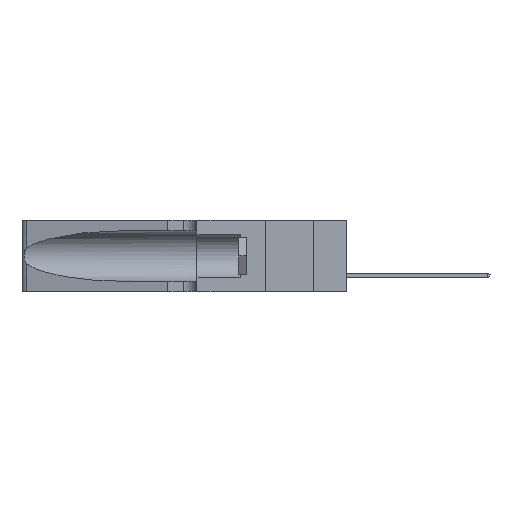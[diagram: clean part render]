
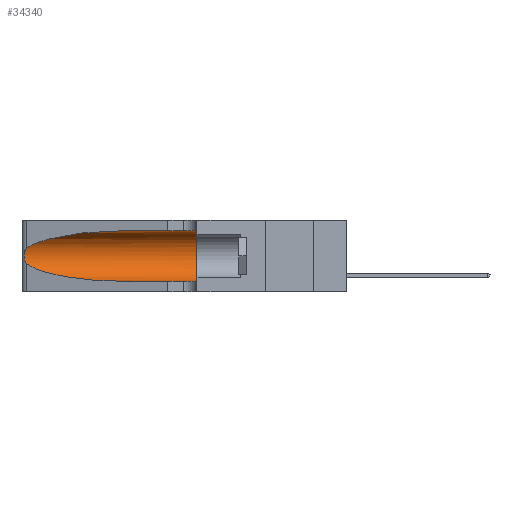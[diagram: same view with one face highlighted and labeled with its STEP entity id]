
A CAD part, left-side view. The second image highlights one B-rep face of the part: STEP entity #34340.
In plain terms, the highlighted cylindrical face has radius 3.308 mm (diameter 6.617 mm), a partial arc.
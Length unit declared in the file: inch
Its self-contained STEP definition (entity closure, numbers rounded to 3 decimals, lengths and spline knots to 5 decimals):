
#323 = EDGE_CURVE ( 'NONE', #18879, #18851, #22355, .T. ) ;
#1879 = ORIENTED_EDGE ( 'NONE', *, *, #11291, .F. ) ;
#2543 = CARTESIAN_POINT ( 'NONE',  ( 0.25555, 1.22993, 0.14849 ) ) ;
#2659 = CARTESIAN_POINT ( 'NONE',  ( 0.2373, 1.15595, 0.08982 ) ) ;
#2706 = CARTESIAN_POINT ( 'NONE',  ( 0.25487, 1.22718, 0.22369 ) ) ;
#3134 = VERTEX_POINT ( 'NONE', #41713 ) ;
#4005 = EDGE_CURVE ( 'NONE', #18851, #28390, #4882, .T. ) ;
#4381 = CARTESIAN_POINT ( 'NONE',  ( 0.26075, 1.23896, 0.178 ) ) ;
#4882 =( BOUNDED_CURVE ( )  B_SPLINE_CURVE ( 3, ( #34687, #2659, #30677, #18717 ),
 .UNSPECIFIED., .F., .F. ) 
 B_SPLINE_CURVE_WITH_KNOTS ( ( 4, 4 ),
 ( 3.44316, 4.71239 ),
 .UNSPECIFIED. ) 
 CURVE ( )  GEOMETRIC_REPRESENTATION_ITEM ( )  RATIONAL_B_SPLINE_CURVE ( ( 1., 0.87, 0.87, 1. ) ) 
 REPRESENTATION_ITEM ( '' )  );
#5112 = LINE ( 'NONE', #31419, #37330 ) ;
#6915 = ORIENTED_EDGE ( 'NONE', *, *, #20891, .T. ) ;
#7603 = CARTESIAN_POINT ( 'NONE',  ( 0.25487, 1.22718, 0.22369 ) ) ;
#7993 = CARTESIAN_POINT ( 'NONE',  ( 0.1305, 1.61858, 0.31525 ) ) ;
#11291 = EDGE_CURVE ( 'NONE', #23974, #41433, #17209, .T. ) ;
#12127 = FACE_OUTER_BOUND ( 'NONE', #50442, .T. ) ;
#14877 = CARTESIAN_POINT ( 'NONE',  ( 0.1305, 0.35, 0.31525 ) ) ;
#15118 = CARTESIAN_POINT ( 'NONE',  ( 0.1305, 0.72297, 0.05475 ) ) ;
#16790 = CARTESIAN_POINT ( 'NONE',  ( 0.26017, 1.23833, 0.17102 ) ) ;
#16837 = EDGE_CURVE ( 'NONE', #3134, #23974, #25311, .T. ) ;
#17209 = CIRCLE ( 'NONE', #35773, 0.13025 ) ;
#18717 = CARTESIAN_POINT ( 'NONE',  ( 0.1305, 0.72297, 0.05475 ) ) ;
#18851 = VERTEX_POINT ( 'NONE', #25180 ) ;
#18879 = VERTEX_POINT ( 'NONE', #41103 ) ;
#19091 = CARTESIAN_POINT ( 'NONE',  ( 0.26075, 1.23896, 0.19203 ) ) ;
#19130 = VECTOR ( 'NONE', #39382, 39.37008 ) ;
#19698 = DIRECTION ( 'NONE',  ( 0., -1., 0. ) ) ;
#20891 = EDGE_CURVE ( 'NONE', #28390, #41433, #5112, .T. ) ;
#21213 = DIRECTION ( 'NONE',  ( 0., 0., 1. ) ) ;
#21400 = CARTESIAN_POINT ( 'NONE',  ( 0.1305, 0.35, 0.185 ) ) ;
#21844 = CARTESIAN_POINT ( 'NONE',  ( 0.25555, 1.22994, 0.2215 ) ) ;
#22230 = CARTESIAN_POINT ( 'NONE',  ( 0.2373, 1.15595, 0.28018 ) ) ;
#22355 = B_SPLINE_CURVE_WITH_KNOTS ( 'NONE', 3,
 ( #7603, #21844, #29826, #35404, #44006, #34300, #19091, #4381, #16790, #46462, #34558, #34379, #2543, #46616 ),
 .UNSPECIFIED., .F., .F.,
 ( 4, 2, 2, 2, 2, 2, 4 ),
 ( 0., 0.00027, 0.00053, 0.00107, 0.0016, 0.00187, 0.00214 ),
 .UNSPECIFIED. ) ;
#22485 = ORIENTED_EDGE ( 'NONE', *, *, #41420, .T. ) ;
#22898 = AXIS2_PLACEMENT_3D ( 'NONE', #35529, #19698, #40472 ) ;
#23974 = VERTEX_POINT ( 'NONE', #14877 ) ;
#25180 = CARTESIAN_POINT ( 'NONE',  ( 0.25487, 1.22718, 0.14631 ) ) ;
#25311 = LINE ( 'NONE', #7993, #19130 ) ;
#25871 = CARTESIAN_POINT ( 'NONE',  ( 0.18966, 0.96281, 0.31525 ) ) ;
#28080 = DIRECTION ( 'NONE',  ( 0., -1., 0. ) ) ;
#28390 = VERTEX_POINT ( 'NONE', #15118 ) ;
#29826 = CARTESIAN_POINT ( 'NONE',  ( 0.25639, 1.23184, 0.21858 ) ) ;
#30677 = CARTESIAN_POINT ( 'NONE',  ( 0.18966, 0.96281, 0.05475 ) ) ;
#31419 = CARTESIAN_POINT ( 'NONE',  ( 0.1305, 1.61858, 0.05475 ) ) ;
#32422 = CARTESIAN_POINT ( 'NONE',  ( 0.1305, 0.72297, 0.31525 ) ) ;
#33847 = CYLINDRICAL_SURFACE ( 'NONE', #22898, 0.13025 ) ;
#34300 = CARTESIAN_POINT ( 'NONE',  ( 0.26018, 1.23835, 0.19895 ) ) ;
#34340 = ADVANCED_FACE ( 'NONE', ( #12127 ), #33847, .F. ) ;
#34379 = CARTESIAN_POINT ( 'NONE',  ( 0.25639, 1.23186, 0.15144 ) ) ;
#34558 = CARTESIAN_POINT ( 'NONE',  ( 0.25789, 1.23486, 0.15765 ) ) ;
#34687 = CARTESIAN_POINT ( 'NONE',  ( 0.25487, 1.22718, 0.14631 ) ) ;
#35404 = CARTESIAN_POINT ( 'NONE',  ( 0.25787, 1.23484, 0.2124 ) ) ;
#35529 = CARTESIAN_POINT ( 'NONE',  ( 0.1305, 1.61858, 0.185 ) ) ;
#35773 = AXIS2_PLACEMENT_3D ( 'NONE', #21400, #40627, #21213 ) ;
#37330 = VECTOR ( 'NONE', #28080, 39.37008 ) ;
#39047 = CARTESIAN_POINT ( 'NONE',  ( 0.1305, 0.35, 0.05475 ) ) ;
#39382 = DIRECTION ( 'NONE',  ( 0., -1., 0. ) ) ;
#40472 = DIRECTION ( 'NONE',  ( 0., 0., -1. ) ) ;
#40627 = DIRECTION ( 'NONE',  ( 0., 1., 0. ) ) ;
#41029 = ORIENTED_EDGE ( 'NONE', *, *, #4005, .T. ) ;
#41103 = CARTESIAN_POINT ( 'NONE',  ( 0.25487, 1.22718, 0.22369 ) ) ;
#41420 = EDGE_CURVE ( 'NONE', #3134, #18879, #50884, .T. ) ;
#41433 = VERTEX_POINT ( 'NONE', #39047 ) ;
#41713 = CARTESIAN_POINT ( 'NONE',  ( 0.1305, 0.72297, 0.31525 ) ) ;
#44006 = CARTESIAN_POINT ( 'NONE',  ( 0.25854, 1.2359, 0.20912 ) ) ;
#45373 = ORIENTED_EDGE ( 'NONE', *, *, #16837, .F. ) ;
#46462 = CARTESIAN_POINT ( 'NONE',  ( 0.25856, 1.23593, 0.16098 ) ) ;
#46616 = CARTESIAN_POINT ( 'NONE',  ( 0.25487, 1.22718, 0.14631 ) ) ;
#48249 = ORIENTED_EDGE ( 'NONE', *, *, #323, .T. ) ;
#50442 = EDGE_LOOP ( 'NONE', ( #22485, #48249, #41029, #6915, #1879, #45373 ) ) ;
#50884 =( BOUNDED_CURVE ( )  B_SPLINE_CURVE ( 3, ( #32422, #25871, #22230, #2706 ),
 .UNSPECIFIED., .F., .F. ) 
 B_SPLINE_CURVE_WITH_KNOTS ( ( 4, 4 ),
 ( 1.5708, 2.84003 ),
 .UNSPECIFIED. ) 
 CURVE ( )  GEOMETRIC_REPRESENTATION_ITEM ( )  RATIONAL_B_SPLINE_CURVE ( ( 1., 0.87, 0.87, 1. ) ) 
 REPRESENTATION_ITEM ( '' )  );
